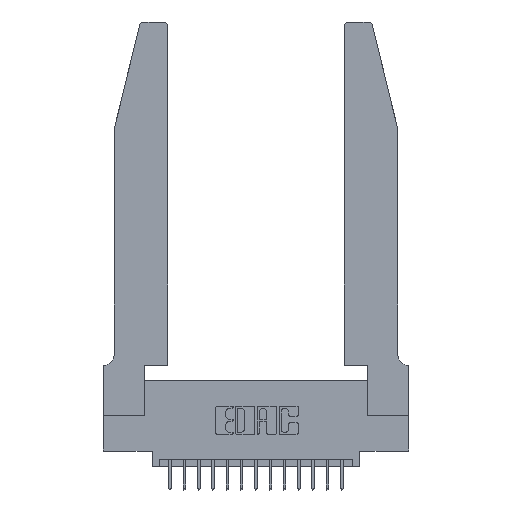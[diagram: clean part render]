
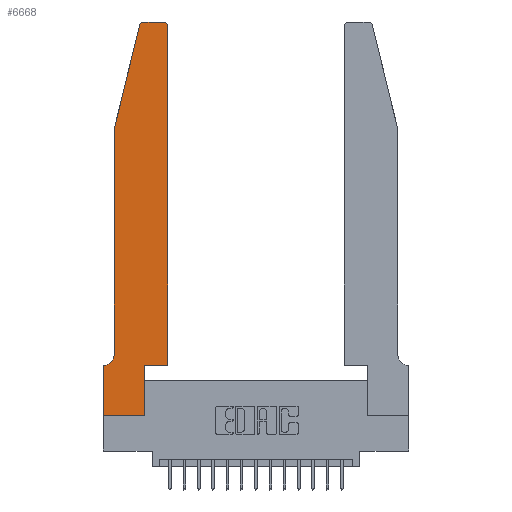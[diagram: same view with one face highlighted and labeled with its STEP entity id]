
A CAD part, top view. The second image highlights one B-rep face of the part: STEP entity #6668.
In plain terms, the highlighted planar face has unit normal (0, 0, 1).
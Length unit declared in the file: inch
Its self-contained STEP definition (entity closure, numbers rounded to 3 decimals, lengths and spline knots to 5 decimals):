
#184 = ORIENTED_EDGE ( 'NONE', *, *, #5774, .T. ) ;
#364 = CARTESIAN_POINT ( 'NONE',  ( 0.284, 2.75, 0.37 ) ) ;
#436 = EDGE_CURVE ( 'NONE', #6035, #4047, #2062, .T. ) ;
#620 = CARTESIAN_POINT ( 'NONE',  ( 0.2605, 2.75, 0.37 ) ) ;
#938 = DIRECTION ( 'NONE',  ( 0., -1., 0. ) ) ;
#1117 = VERTEX_POINT ( 'NONE', #7116 ) ;
#1135 = CARTESIAN_POINT ( 'NONE',  ( 0.0755, 2., 0.37 ) ) ;
#1303 = CARTESIAN_POINT ( 'NONE',  ( 0.2865, 0.35, 0.37 ) ) ;
#1361 = CARTESIAN_POINT ( 'NONE',  ( 0.0055, 0.42, 0.37 ) ) ;
#1470 = ORIENTED_EDGE ( 'NONE', *, *, #10999, .T. ) ;
#1686 = AXIS2_PLACEMENT_3D ( 'NONE', #1361, #4298, #13065 ) ;
#2062 = LINE ( 'NONE', #2658, #17264 ) ;
#2426 = ORIENTED_EDGE ( 'NONE', *, *, #16920, .T. ) ;
#2658 = CARTESIAN_POINT ( 'NONE',  ( 0.0755, 0.35, 0.37 ) ) ;
#3028 = LINE ( 'NONE', #15673, #9451 ) ;
#3254 = EDGE_CURVE ( 'NONE', #13610, #13582, #13543, .T. ) ;
#3263 = LINE ( 'NONE', #620, #13397 ) ;
#3461 = ORIENTED_EDGE ( 'NONE', *, *, #10288, .T. ) ;
#3737 = VERTEX_POINT ( 'NONE', #364 ) ;
#3739 = VERTEX_POINT ( 'NONE', #12015 ) ;
#3812 = PLANE ( 'NONE',  #12938 ) ;
#4047 = VERTEX_POINT ( 'NONE', #10220 ) ;
#4124 = LINE ( 'NONE', #12460, #8510 ) ;
#4298 = DIRECTION ( 'NONE',  ( 0., 0., -1. ) ) ;
#4314 = EDGE_LOOP ( 'NONE', ( #7240, #16233, #7709, #184, #2426, #14574, #14931, #5834, #16008, #1470, #7428, #3461 ) ) ;
#4325 = AXIS2_PLACEMENT_3D ( 'NONE', #5430, #11441, #15827 ) ;
#4515 = CIRCLE ( 'NONE', #4325, 0.03 ) ;
#4534 = CARTESIAN_POINT ( 'NONE',  ( 0.4505, 0.35, 0.37 ) ) ;
#4677 = VERTEX_POINT ( 'NONE', #11171 ) ;
#4907 = DIRECTION ( 'NONE',  ( 1., 0., 0. ) ) ;
#5310 = VERTEX_POINT ( 'NONE', #7913 ) ;
#5430 = CARTESIAN_POINT ( 'NONE',  ( 0.284, 2.72, 0.37 ) ) ;
#5774 = EDGE_CURVE ( 'NONE', #3739, #1117, #15537, .T. ) ;
#5834 = ORIENTED_EDGE ( 'NONE', *, *, #16454, .T. ) ;
#5860 = DIRECTION ( 'NONE',  ( 0., 0., 1. ) ) ;
#5923 = CARTESIAN_POINT ( 'NONE',  ( 0.4505, 0.35, 0.37 ) ) ;
#6035 = VERTEX_POINT ( 'NONE', #8986 ) ;
#6295 = VECTOR ( 'NONE', #938, 39.37008 ) ;
#6668 = ADVANCED_FACE ( 'NONE', ( #11805 ), #3812, .T. ) ;
#7116 = CARTESIAN_POINT ( 'NONE',  ( 0.0755, 0.42, 0.37 ) ) ;
#7240 = ORIENTED_EDGE ( 'NONE', *, *, #14601, .T. ) ;
#7411 = CARTESIAN_POINT ( 'NONE',  ( 0., 0., 0.37 ) ) ;
#7428 = ORIENTED_EDGE ( 'NONE', *, *, #7446, .T. ) ;
#7446 = EDGE_CURVE ( 'NONE', #4677, #12265, #8190, .T. ) ;
#7709 = ORIENTED_EDGE ( 'NONE', *, *, #15840, .T. ) ;
#7820 = CIRCLE ( 'NONE', #12967, 0.03 ) ;
#7913 = CARTESIAN_POINT ( 'NONE',  ( 0., 0., 0.37 ) ) ;
#8189 = CARTESIAN_POINT ( 'NONE',  ( 0., 0.35, 0.37 ) ) ;
#8190 = LINE ( 'NONE', #4534, #14820 ) ;
#8276 = DIRECTION ( 'NONE',  ( 0., -1., 0. ) ) ;
#8452 = CARTESIAN_POINT ( 'NONE',  ( 0.4205, 2.72, 0.37 ) ) ;
#8486 = LINE ( 'NONE', #5923, #15863 ) ;
#8510 = VECTOR ( 'NONE', #12389, 39.37008 ) ;
#8986 = CARTESIAN_POINT ( 'NONE',  ( 0.0055, 0.35, 0.37 ) ) ;
#9451 = VECTOR ( 'NONE', #8276, 39.37008 ) ;
#10220 = CARTESIAN_POINT ( 'NONE',  ( 0., 0.35, 0.37 ) ) ;
#10288 = EDGE_CURVE ( 'NONE', #12265, #13692, #7820, .T. ) ;
#10295 = DIRECTION ( 'NONE',  ( 1., 0., 0. ) ) ;
#10349 = CARTESIAN_POINT ( 'NONE',  ( 0.4205, 2.75, 0.37 ) ) ;
#10599 = CARTESIAN_POINT ( 'NONE',  ( 0.2865, 0.35, 0.37 ) ) ;
#10905 = DIRECTION ( 'NONE',  ( -1., 0., 0. ) ) ;
#10999 = EDGE_CURVE ( 'NONE', #13582, #4677, #8486, .T. ) ;
#11171 = CARTESIAN_POINT ( 'NONE',  ( 0.4505, 0.35, 0.37 ) ) ;
#11441 = DIRECTION ( 'NONE',  ( 0., 0., 1. ) ) ;
#11459 = CIRCLE ( 'NONE', #1686, 0.07 ) ;
#11805 = FACE_OUTER_BOUND ( 'NONE', #4314, .T. ) ;
#11910 = DIRECTION ( 'NONE',  ( 1., 0., 0. ) ) ;
#12015 = CARTESIAN_POINT ( 'NONE',  ( 0.0755, 2., 0.37 ) ) ;
#12265 = VERTEX_POINT ( 'NONE', #12802 ) ;
#12389 = DIRECTION ( 'NONE',  ( -0.239, -0.971, 0. ) ) ;
#12460 = CARTESIAN_POINT ( 'NONE',  ( 0.0755, 2., 0.37 ) ) ;
#12802 = CARTESIAN_POINT ( 'NONE',  ( 0.4505, 2.72, 0.37 ) ) ;
#12819 = CARTESIAN_POINT ( 'NONE',  ( 0.2865, 0., 0.37 ) ) ;
#12938 = AXIS2_PLACEMENT_3D ( 'NONE', #8189, #14624, #11910 ) ;
#12967 = AXIS2_PLACEMENT_3D ( 'NONE', #8452, #5860, #10295 ) ;
#13065 = DIRECTION ( 'NONE',  ( -1., 0., 0. ) ) ;
#13397 = VECTOR ( 'NONE', #10905, 39.37008 ) ;
#13543 = LINE ( 'NONE', #10599, #16553 ) ;
#13582 = VERTEX_POINT ( 'NONE', #1303 ) ;
#13610 = VERTEX_POINT ( 'NONE', #12819 ) ;
#13692 = VERTEX_POINT ( 'NONE', #10349 ) ;
#13772 = LINE ( 'NONE', #7411, #16787 ) ;
#14574 = ORIENTED_EDGE ( 'NONE', *, *, #436, .T. ) ;
#14601 = EDGE_CURVE ( 'NONE', #13692, #3737, #3263, .T. ) ;
#14624 = DIRECTION ( 'NONE',  ( 0., 0., 1. ) ) ;
#14820 = VECTOR ( 'NONE', #17878, 39.37008 ) ;
#14931 = ORIENTED_EDGE ( 'NONE', *, *, #14953, .T. ) ;
#14953 = EDGE_CURVE ( 'NONE', #4047, #5310, #3028, .T. ) ;
#15117 = DIRECTION ( 'NONE',  ( 0., 1., 0. ) ) ;
#15193 = DIRECTION ( 'NONE',  ( 1., 0., 0. ) ) ;
#15339 = VERTEX_POINT ( 'NONE', #15397 ) ;
#15397 = CARTESIAN_POINT ( 'NONE',  ( 0.25487, 2.72718, 0.37 ) ) ;
#15537 = LINE ( 'NONE', #1135, #6295 ) ;
#15673 = CARTESIAN_POINT ( 'NONE',  ( 0., 0., 0.37 ) ) ;
#15827 = DIRECTION ( 'NONE',  ( 1., 0., 0. ) ) ;
#15840 = EDGE_CURVE ( 'NONE', #15339, #3739, #4124, .T. ) ;
#15863 = VECTOR ( 'NONE', #15193, 39.37008 ) ;
#16008 = ORIENTED_EDGE ( 'NONE', *, *, #3254, .T. ) ;
#16233 = ORIENTED_EDGE ( 'NONE', *, *, #17508, .T. ) ;
#16454 = EDGE_CURVE ( 'NONE', #5310, #13610, #13772, .T. ) ;
#16553 = VECTOR ( 'NONE', #15117, 39.37008 ) ;
#16787 = VECTOR ( 'NONE', #4907, 39.37008 ) ;
#16920 = EDGE_CURVE ( 'NONE', #1117, #6035, #11459, .T. ) ;
#17264 = VECTOR ( 'NONE', #17524, 39.37008 ) ;
#17508 = EDGE_CURVE ( 'NONE', #3737, #15339, #4515, .T. ) ;
#17524 = DIRECTION ( 'NONE',  ( -1., 0., 0. ) ) ;
#17878 = DIRECTION ( 'NONE',  ( 0., 1., 0. ) ) ;
